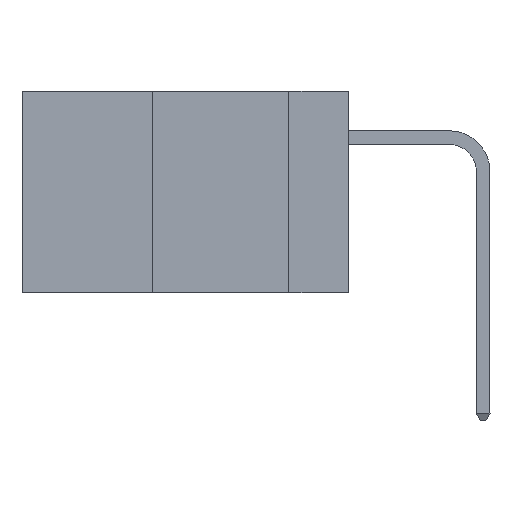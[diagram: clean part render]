
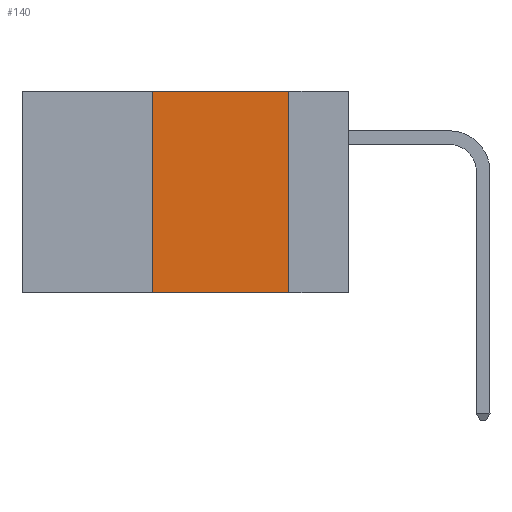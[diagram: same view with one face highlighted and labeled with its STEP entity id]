
A CAD part, left-side view. The second image highlights one B-rep face of the part: STEP entity #140.
In plain terms, the highlighted planar face has unit normal (-1, 0, 0).
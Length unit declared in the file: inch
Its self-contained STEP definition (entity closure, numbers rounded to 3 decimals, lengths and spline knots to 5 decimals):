
#140 = ADVANCED_FACE ( 'NONE', ( #15152 ), #12039, .F. ) ;
#344 = ORIENTED_EDGE ( 'NONE', *, *, #15162, .F. ) ;
#585 = VECTOR ( 'NONE', #1914, 39.37008 ) ;
#649 = EDGE_CURVE ( 'NONE', #12388, #2228, #5351, .T. ) ;
#860 = VECTOR ( 'NONE', #6616, 39.37008 ) ;
#1660 = CARTESIAN_POINT ( 'NONE',  ( 0., 0.11, 0. ) ) ;
#1914 = DIRECTION ( 'NONE',  ( 0., 0., 1. ) ) ;
#2032 = CARTESIAN_POINT ( 'NONE',  ( 0., 0.11, 0. ) ) ;
#2228 = VERTEX_POINT ( 'NONE', #1660 ) ;
#3381 = CARTESIAN_POINT ( 'NONE',  ( 0., 0.36, 0. ) ) ;
#3551 = CARTESIAN_POINT ( 'NONE',  ( 0., 0.6, 0. ) ) ;
#3597 = ORIENTED_EDGE ( 'NONE', *, *, #649, .F. ) ;
#3895 = AXIS2_PLACEMENT_3D ( 'NONE', #3551, #4730, #17967 ) ;
#4730 = DIRECTION ( 'NONE',  ( 1., 0., 0. ) ) ;
#5351 = LINE ( 'NONE', #12853, #5371 ) ;
#5371 = VECTOR ( 'NONE', #17415, 39.37008 ) ;
#6616 = DIRECTION ( 'NONE',  ( 0., 0., -1. ) ) ;
#6837 = EDGE_CURVE ( 'NONE', #9149, #14932, #10371, .T. ) ;
#9149 = VERTEX_POINT ( 'NONE', #17871 ) ;
#9450 = LINE ( 'NONE', #2032, #860 ) ;
#9451 = ORIENTED_EDGE ( 'NONE', *, *, #6837, .T. ) ;
#10000 = VECTOR ( 'NONE', #19233, 39.37008 ) ;
#10371 = LINE ( 'NONE', #14758, #10000 ) ;
#10804 = LINE ( 'NONE', #3381, #585 ) ;
#11767 = CARTESIAN_POINT ( 'NONE',  ( 0., 0.36, 0. ) ) ;
#12039 = PLANE ( 'NONE',  #3895 ) ;
#12071 = EDGE_CURVE ( 'NONE', #2228, #14932, #9450, .T. ) ;
#12388 = VERTEX_POINT ( 'NONE', #11767 ) ;
#12853 = CARTESIAN_POINT ( 'NONE',  ( 0., 0.6, 0. ) ) ;
#14167 = ORIENTED_EDGE ( 'NONE', *, *, #12071, .F. ) ;
#14758 = CARTESIAN_POINT ( 'NONE',  ( 0., 0.6, -0.37 ) ) ;
#14932 = VERTEX_POINT ( 'NONE', #19184 ) ;
#15152 = FACE_OUTER_BOUND ( 'NONE', #18251, .T. ) ;
#15162 = EDGE_CURVE ( 'NONE', #9149, #12388, #10804, .T. ) ;
#17415 = DIRECTION ( 'NONE',  ( 0., -1., 0. ) ) ;
#17871 = CARTESIAN_POINT ( 'NONE',  ( 0., 0.36, -0.37 ) ) ;
#17967 = DIRECTION ( 'NONE',  ( 0., 0., -1. ) ) ;
#18251 = EDGE_LOOP ( 'NONE', ( #14167, #3597, #344, #9451 ) ) ;
#19184 = CARTESIAN_POINT ( 'NONE',  ( 0., 0.11, -0.37 ) ) ;
#19233 = DIRECTION ( 'NONE',  ( 0., -1., 0. ) ) ;
